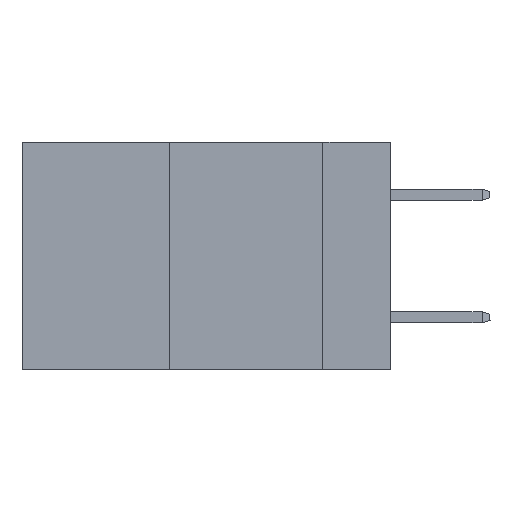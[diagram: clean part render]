
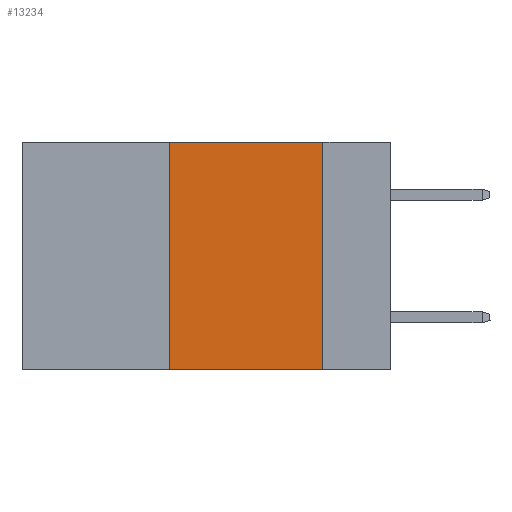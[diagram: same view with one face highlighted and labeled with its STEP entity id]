
A CAD part, left-side view. The second image highlights one B-rep face of the part: STEP entity #13234.
In plain terms, the highlighted planar face has unit normal (-1, 0, 0).
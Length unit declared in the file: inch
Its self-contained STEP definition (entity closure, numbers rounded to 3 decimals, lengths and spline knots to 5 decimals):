
#83 = DIRECTION ( 'NONE',  ( 1., 0., 0. ) ) ;
#305 = CARTESIAN_POINT ( 'NONE',  ( 0., 0.36, 0. ) ) ;
#1734 = CARTESIAN_POINT ( 'NONE',  ( 0., 0.11, 0. ) ) ;
#2641 = VERTEX_POINT ( 'NONE', #8509 ) ;
#2946 = VERTEX_POINT ( 'NONE', #13800 ) ;
#4839 = EDGE_CURVE ( 'NONE', #2641, #11192, #6952, .T. ) ;
#5305 = LINE ( 'NONE', #11850, #13053 ) ;
#5414 = VECTOR ( 'NONE', #8643, 39.37008 ) ;
#6263 = ORIENTED_EDGE ( 'NONE', *, *, #4839, .F. ) ;
#6465 = EDGE_CURVE ( 'NONE', #11192, #13284, #15267, .T. ) ;
#6952 = LINE ( 'NONE', #305, #14625 ) ;
#7150 = VECTOR ( 'NONE', #16736, 39.37008 ) ;
#7337 = FACE_OUTER_BOUND ( 'NONE', #12152, .T. ) ;
#7586 = CARTESIAN_POINT ( 'NONE',  ( 0., 0.6, 0. ) ) ;
#8076 = EDGE_CURVE ( 'NONE', #13284, #2946, #5305, .T. ) ;
#8495 = ORIENTED_EDGE ( 'NONE', *, *, #6465, .F. ) ;
#8509 = CARTESIAN_POINT ( 'NONE',  ( 0., 0.36, -0.37 ) ) ;
#8643 = DIRECTION ( 'NONE',  ( 0., -1., 0. ) ) ;
#9221 = ORIENTED_EDGE ( 'NONE', *, *, #11114, .T. ) ;
#9507 = PLANE ( 'NONE',  #15920 ) ;
#9573 = CARTESIAN_POINT ( 'NONE',  ( 0., 0.6, 0. ) ) ;
#10066 = LINE ( 'NONE', #19211, #5414 ) ;
#11094 = DIRECTION ( 'NONE',  ( 0., 0., -1. ) ) ;
#11114 = EDGE_CURVE ( 'NONE', #2641, #2946, #10066, .T. ) ;
#11192 = VERTEX_POINT ( 'NONE', #14891 ) ;
#11850 = CARTESIAN_POINT ( 'NONE',  ( 0., 0.11, 0. ) ) ;
#12152 = EDGE_LOOP ( 'NONE', ( #17766, #8495, #6263, #9221 ) ) ;
#12835 = DIRECTION ( 'NONE',  ( 0., 0., 1. ) ) ;
#13053 = VECTOR ( 'NONE', #14918, 39.37008 ) ;
#13234 = ADVANCED_FACE ( 'NONE', ( #7337 ), #9507, .F. ) ;
#13284 = VERTEX_POINT ( 'NONE', #1734 ) ;
#13800 = CARTESIAN_POINT ( 'NONE',  ( 0., 0.11, -0.37 ) ) ;
#14625 = VECTOR ( 'NONE', #12835, 39.37008 ) ;
#14891 = CARTESIAN_POINT ( 'NONE',  ( 0., 0.36, 0. ) ) ;
#14918 = DIRECTION ( 'NONE',  ( 0., 0., -1. ) ) ;
#15267 = LINE ( 'NONE', #7586, #7150 ) ;
#15920 = AXIS2_PLACEMENT_3D ( 'NONE', #9573, #83, #11094 ) ;
#16736 = DIRECTION ( 'NONE',  ( 0., -1., 0. ) ) ;
#17766 = ORIENTED_EDGE ( 'NONE', *, *, #8076, .F. ) ;
#19211 = CARTESIAN_POINT ( 'NONE',  ( 0., 0.6, -0.37 ) ) ;
